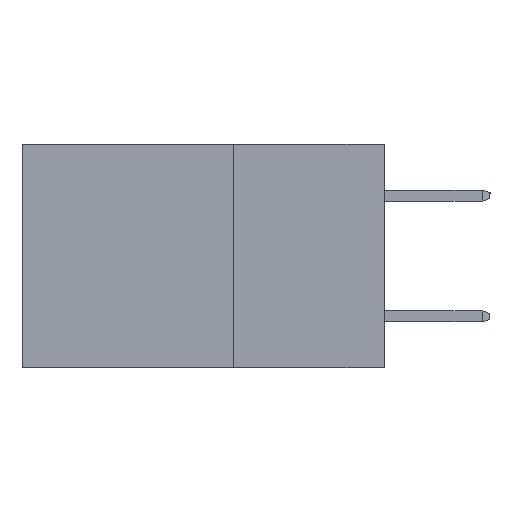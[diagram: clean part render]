
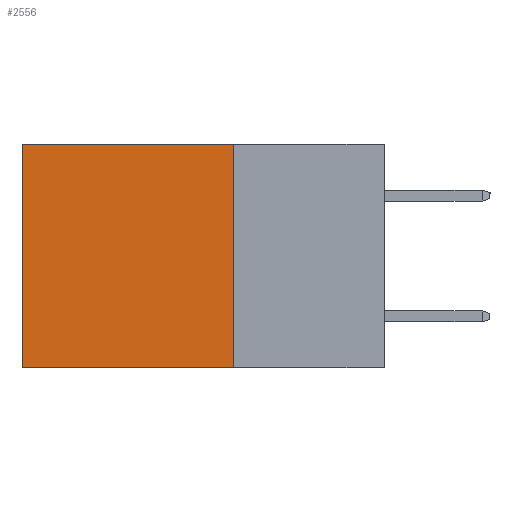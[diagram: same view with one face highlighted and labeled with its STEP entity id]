
A CAD part, left-side view. The second image highlights one B-rep face of the part: STEP entity #2556.
In plain terms, the highlighted planar face has unit normal (-1, 0, 0).
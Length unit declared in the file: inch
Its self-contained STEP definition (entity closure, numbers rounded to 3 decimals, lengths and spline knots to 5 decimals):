
#221 = LINE ( 'NONE', #998, #6106 ) ;
#314 = ORIENTED_EDGE ( 'NONE', *, *, #5743, .F. ) ;
#383 = VERTEX_POINT ( 'NONE', #3044 ) ;
#771 = ORIENTED_EDGE ( 'NONE', *, *, #9508, .F. ) ;
#998 = CARTESIAN_POINT ( 'NONE',  ( 0.2615, 0.25, -0.37 ) ) ;
#1143 = EDGE_CURVE ( 'NONE', #1464, #1605, #2231, .T. ) ;
#1164 = DIRECTION ( 'NONE',  ( 0., 0., -1. ) ) ;
#1401 = LINE ( 'NONE', #2868, #7905 ) ;
#1464 = VERTEX_POINT ( 'NONE', #6005 ) ;
#1488 = DIRECTION ( 'NONE',  ( 0., 0., -1. ) ) ;
#1605 = VERTEX_POINT ( 'NONE', #6323 ) ;
#1927 = DIRECTION ( 'NONE',  ( 1., 0., 0. ) ) ;
#2231 = LINE ( 'NONE', #8973, #2834 ) ;
#2246 = AXIS2_PLACEMENT_3D ( 'NONE', #9363, #1927, #4138 ) ;
#2420 = DIRECTION ( 'NONE',  ( 0., 1., 0. ) ) ;
#2556 = ADVANCED_FACE ( 'NONE', ( #4091 ), #5510, .F. ) ;
#2779 = VECTOR ( 'NONE', #1164, 39.37008 ) ;
#2834 = VECTOR ( 'NONE', #5224, 39.37008 ) ;
#2868 = CARTESIAN_POINT ( 'NONE',  ( 0.2615, 0.25, -0.37 ) ) ;
#3044 = CARTESIAN_POINT ( 'NONE',  ( 0.2615, 0.25, -0.37 ) ) ;
#4053 = EDGE_CURVE ( 'NONE', #1605, #8074, #4102, .T. ) ;
#4091 = FACE_OUTER_BOUND ( 'NONE', #7266, .T. ) ;
#4102 = LINE ( 'NONE', #4885, #2779 ) ;
#4138 = DIRECTION ( 'NONE',  ( 0., 0., -1. ) ) ;
#4345 = ORIENTED_EDGE ( 'NONE', *, *, #4053, .T. ) ;
#4885 = CARTESIAN_POINT ( 'NONE',  ( 0.2615, 0.6, -0.37 ) ) ;
#5224 = DIRECTION ( 'NONE',  ( 0., 1., 0. ) ) ;
#5510 = PLANE ( 'NONE',  #2246 ) ;
#5743 = EDGE_CURVE ( 'NONE', #1464, #383, #1401, .T. ) ;
#6005 = CARTESIAN_POINT ( 'NONE',  ( 0.2615, 0.25, 0. ) ) ;
#6106 = VECTOR ( 'NONE', #2420, 39.37008 ) ;
#6323 = CARTESIAN_POINT ( 'NONE',  ( 0.2615, 0.6, 0. ) ) ;
#7266 = EDGE_LOOP ( 'NONE', ( #4345, #771, #314, #8772 ) ) ;
#7905 = VECTOR ( 'NONE', #1488, 39.37008 ) ;
#8074 = VERTEX_POINT ( 'NONE', #9051 ) ;
#8772 = ORIENTED_EDGE ( 'NONE', *, *, #1143, .T. ) ;
#8973 = CARTESIAN_POINT ( 'NONE',  ( 0.2615, 0.25, 0. ) ) ;
#9051 = CARTESIAN_POINT ( 'NONE',  ( 0.2615, 0.6, -0.37 ) ) ;
#9363 = CARTESIAN_POINT ( 'NONE',  ( 0.2615, 0.25, -0.37 ) ) ;
#9508 = EDGE_CURVE ( 'NONE', #383, #8074, #221, .T. ) ;
